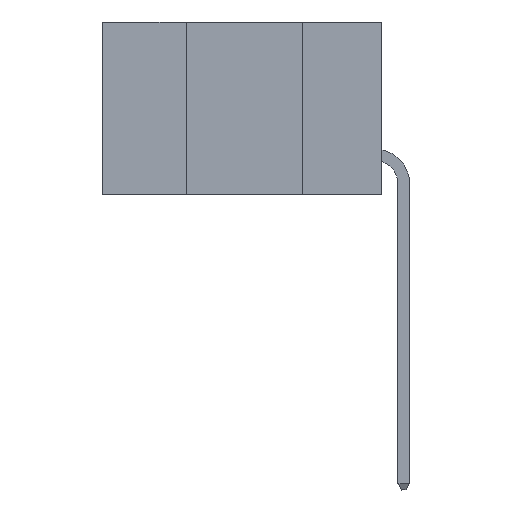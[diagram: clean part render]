
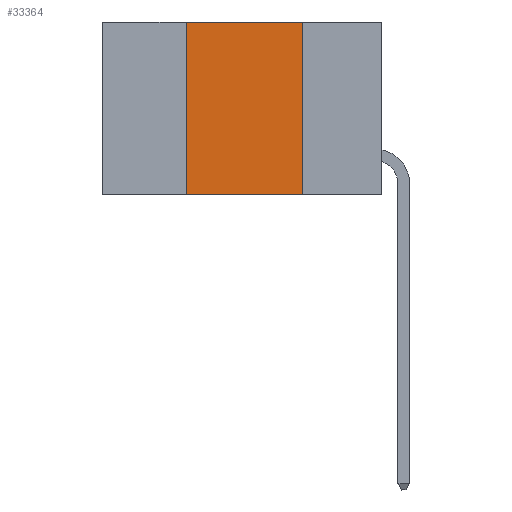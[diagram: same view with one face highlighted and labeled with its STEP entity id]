
A CAD part, left-side view. The second image highlights one B-rep face of the part: STEP entity #33364.
In plain terms, the highlighted planar face has unit normal (-1, 0, 0).
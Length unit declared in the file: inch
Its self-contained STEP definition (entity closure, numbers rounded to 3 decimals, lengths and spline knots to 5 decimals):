
#2505 = EDGE_CURVE ( 'NONE', #3442, #40562, #16225, .T. ) ;
#3442 = VERTEX_POINT ( 'NONE', #22945 ) ;
#4816 = LINE ( 'NONE', #26566, #19669 ) ;
#5742 = DIRECTION ( 'NONE',  ( 0., 0., -1. ) ) ;
#6041 = DIRECTION ( 'NONE',  ( 0., -1., 0. ) ) ;
#8954 = DIRECTION ( 'NONE',  ( 0., 0., -1. ) ) ;
#10687 = AXIS2_PLACEMENT_3D ( 'NONE', #36986, #44355, #5742 ) ;
#11513 = ORIENTED_EDGE ( 'NONE', *, *, #11935, .T. ) ;
#11935 = EDGE_CURVE ( 'NONE', #17775, #23840, #24820, .T. ) ;
#12215 = VECTOR ( 'NONE', #6041, 39.37008 ) ;
#13088 = PLANE ( 'NONE',  #10687 ) ;
#16225 = LINE ( 'NONE', #45336, #33729 ) ;
#17400 = CARTESIAN_POINT ( 'NONE',  ( 0., 0.42, -0.37 ) ) ;
#17775 = VERTEX_POINT ( 'NONE', #17400 ) ;
#18363 = ORIENTED_EDGE ( 'NONE', *, *, #22553, .F. ) ;
#19669 = VECTOR ( 'NONE', #8954, 39.37008 ) ;
#20911 = FACE_OUTER_BOUND ( 'NONE', #21036, .T. ) ;
#21036 = EDGE_LOOP ( 'NONE', ( #43561, #35204, #18363, #11513 ) ) ;
#22553 = EDGE_CURVE ( 'NONE', #17775, #3442, #44144, .T. ) ;
#22658 = CARTESIAN_POINT ( 'NONE',  ( 0., 0.17, -0.37 ) ) ;
#22945 = CARTESIAN_POINT ( 'NONE',  ( 0., 0.42, 0. ) ) ;
#23509 = CARTESIAN_POINT ( 'NONE',  ( 0., 0.6, -0.37 ) ) ;
#23840 = VERTEX_POINT ( 'NONE', #22658 ) ;
#24820 = LINE ( 'NONE', #23509, #12215 ) ;
#26566 = CARTESIAN_POINT ( 'NONE',  ( 0., 0.17, 0. ) ) ;
#27725 = CARTESIAN_POINT ( 'NONE',  ( 0., 0.17, 0. ) ) ;
#27981 = EDGE_CURVE ( 'NONE', #40562, #23840, #4816, .T. ) ;
#30772 = DIRECTION ( 'NONE',  ( 0., -1., 0. ) ) ;
#33329 = DIRECTION ( 'NONE',  ( 0., 0., 1. ) ) ;
#33364 = ADVANCED_FACE ( 'NONE', ( #20911 ), #13088, .F. ) ;
#33729 = VECTOR ( 'NONE', #30772, 39.37008 ) ;
#35204 = ORIENTED_EDGE ( 'NONE', *, *, #2505, .F. ) ;
#36986 = CARTESIAN_POINT ( 'NONE',  ( 0., 0.6, 0. ) ) ;
#36989 = VECTOR ( 'NONE', #33329, 39.37008 ) ;
#40513 = CARTESIAN_POINT ( 'NONE',  ( 0., 0.42, 0. ) ) ;
#40562 = VERTEX_POINT ( 'NONE', #27725 ) ;
#43561 = ORIENTED_EDGE ( 'NONE', *, *, #27981, .F. ) ;
#44144 = LINE ( 'NONE', #40513, #36989 ) ;
#44355 = DIRECTION ( 'NONE',  ( 1., 0., 0. ) ) ;
#45336 = CARTESIAN_POINT ( 'NONE',  ( 0., 0.6, 0. ) ) ;
